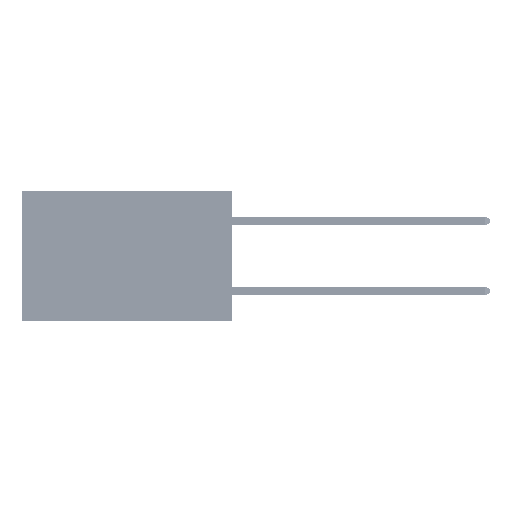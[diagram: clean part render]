
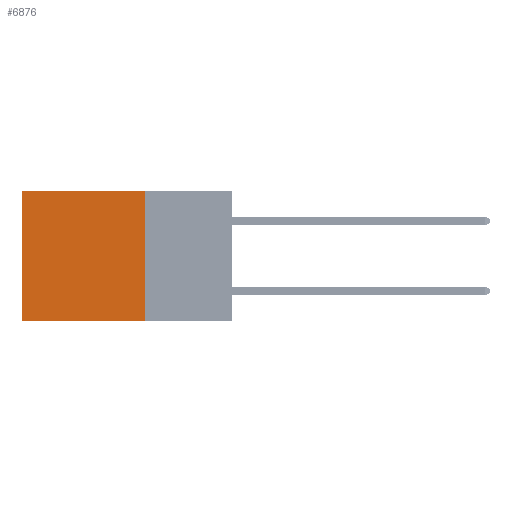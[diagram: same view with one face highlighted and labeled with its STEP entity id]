
A CAD part, left-side view. The second image highlights one B-rep face of the part: STEP entity #6876.
In plain terms, the highlighted planar face has unit normal (-1, 0, 0).
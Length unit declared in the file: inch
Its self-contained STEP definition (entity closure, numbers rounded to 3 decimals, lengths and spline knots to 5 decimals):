
#1107 = ORIENTED_EDGE ( 'NONE', *, *, #27212, .T. ) ;
#2145 = VERTEX_POINT ( 'NONE', #23405 ) ;
#2488 = DIRECTION ( 'NONE',  ( 0., 1., 0. ) ) ;
#4286 = CARTESIAN_POINT ( 'NONE',  ( 0.2875, 0.6, -0.37 ) ) ;
#4916 = LINE ( 'NONE', #26009, #26006 ) ;
#5388 = LINE ( 'NONE', #49554, #41816 ) ;
#6876 = ADVANCED_FACE ( 'NONE', ( #33464 ), #17310, .F. ) ;
#7658 = ORIENTED_EDGE ( 'NONE', *, *, #32280, .F. ) ;
#7890 = VERTEX_POINT ( 'NONE', #4286 ) ;
#9725 = DIRECTION ( 'NONE',  ( 0., 0., -1. ) ) ;
#11820 = EDGE_LOOP ( 'NONE', ( #31947, #49413, #7658, #1107 ) ) ;
#12761 = VERTEX_POINT ( 'NONE', #28592 ) ;
#17277 = VECTOR ( 'NONE', #49902, 39.37008 ) ;
#17310 = PLANE ( 'NONE',  #19004 ) ;
#17491 = DIRECTION ( 'NONE',  ( 1., 0., 0. ) ) ;
#17636 = LINE ( 'NONE', #26932, #25337 ) ;
#19004 = AXIS2_PLACEMENT_3D ( 'NONE', #30003, #17491, #45839 ) ;
#23405 = CARTESIAN_POINT ( 'NONE',  ( 0.2875, 0.25, 0. ) ) ;
#25337 = VECTOR ( 'NONE', #2488, 39.37008 ) ;
#26006 = VECTOR ( 'NONE', #9725, 39.37008 ) ;
#26009 = CARTESIAN_POINT ( 'NONE',  ( 0.2875, 0.6, 0. ) ) ;
#26932 = CARTESIAN_POINT ( 'NONE',  ( 0.2875, 0.25, -0.37 ) ) ;
#27212 = EDGE_CURVE ( 'NONE', #2145, #28155, #5388, .T. ) ;
#28155 = VERTEX_POINT ( 'NONE', #47128 ) ;
#28592 = CARTESIAN_POINT ( 'NONE',  ( 0.2875, 0.25, -0.37 ) ) ;
#30003 = CARTESIAN_POINT ( 'NONE',  ( 0.2875, 0.25, 0. ) ) ;
#30116 = LINE ( 'NONE', #33513, #17277 ) ;
#31947 = ORIENTED_EDGE ( 'NONE', *, *, #47833, .T. ) ;
#32280 = EDGE_CURVE ( 'NONE', #2145, #12761, #30116, .T. ) ;
#33464 = FACE_OUTER_BOUND ( 'NONE', #11820, .T. ) ;
#33513 = CARTESIAN_POINT ( 'NONE',  ( 0.2875, 0.25, 0. ) ) ;
#41816 = VECTOR ( 'NONE', #48851, 39.37008 ) ;
#45839 = DIRECTION ( 'NONE',  ( 0., 0., -1. ) ) ;
#47091 = EDGE_CURVE ( 'NONE', #12761, #7890, #17636, .T. ) ;
#47128 = CARTESIAN_POINT ( 'NONE',  ( 0.2875, 0.6, 0. ) ) ;
#47833 = EDGE_CURVE ( 'NONE', #28155, #7890, #4916, .T. ) ;
#48851 = DIRECTION ( 'NONE',  ( 0., 1., 0. ) ) ;
#49413 = ORIENTED_EDGE ( 'NONE', *, *, #47091, .F. ) ;
#49554 = CARTESIAN_POINT ( 'NONE',  ( 0.2875, 0.25, 0. ) ) ;
#49902 = DIRECTION ( 'NONE',  ( 0., 0., -1. ) ) ;
